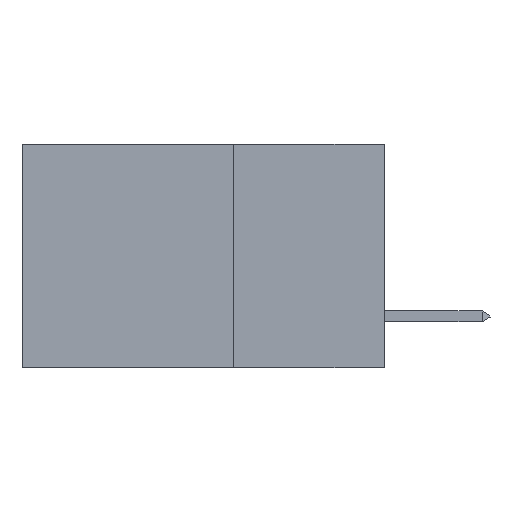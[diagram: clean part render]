
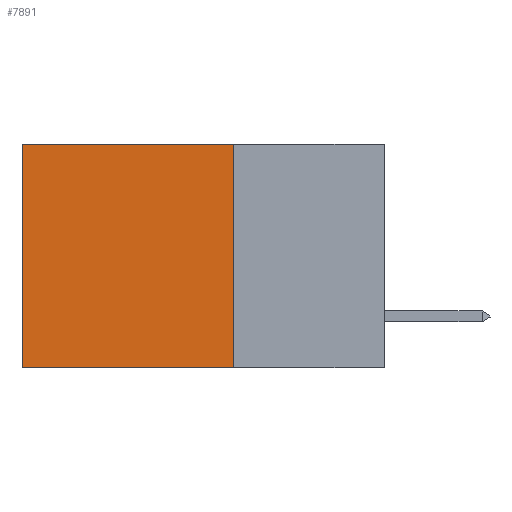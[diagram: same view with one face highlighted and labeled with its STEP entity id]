
A CAD part, left-side view. The second image highlights one B-rep face of the part: STEP entity #7891.
In plain terms, the highlighted planar face has unit normal (-1, 0, 0).
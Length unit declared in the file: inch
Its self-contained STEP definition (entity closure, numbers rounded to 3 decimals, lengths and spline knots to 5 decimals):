
#232 = ORIENTED_EDGE ( 'NONE', *, *, #8652, .T. ) ;
#660 = VERTEX_POINT ( 'NONE', #7267 ) ;
#1251 = EDGE_CURVE ( 'NONE', #660, #13368, #4878, .T. ) ;
#1410 = CARTESIAN_POINT ( 'NONE',  ( 0.2875, 0.25, 0. ) ) ;
#1565 = VECTOR ( 'NONE', #8554, 39.37008 ) ;
#3759 = ORIENTED_EDGE ( 'NONE', *, *, #11474, .T. ) ;
#3905 = VERTEX_POINT ( 'NONE', #6622 ) ;
#4120 = DIRECTION ( 'NONE',  ( 0., 0., -1. ) ) ;
#4446 = VECTOR ( 'NONE', #12484, 39.37008 ) ;
#4835 = LINE ( 'NONE', #7231, #4446 ) ;
#4878 = LINE ( 'NONE', #7297, #1565 ) ;
#4925 = VECTOR ( 'NONE', #14287, 39.37008 ) ;
#5098 = ORIENTED_EDGE ( 'NONE', *, *, #14194, .F. ) ;
#6283 = AXIS2_PLACEMENT_3D ( 'NONE', #7905, #9065, #4120 ) ;
#6622 = CARTESIAN_POINT ( 'NONE',  ( 0.2875, 0.25, 0. ) ) ;
#7231 = CARTESIAN_POINT ( 'NONE',  ( 0.2875, 0.25, 0. ) ) ;
#7267 = CARTESIAN_POINT ( 'NONE',  ( 0.2875, 0.25, -0.37 ) ) ;
#7297 = CARTESIAN_POINT ( 'NONE',  ( 0.2875, 0.25, -0.37 ) ) ;
#7891 = ADVANCED_FACE ( 'NONE', ( #11347 ), #15352, .F. ) ;
#7905 = CARTESIAN_POINT ( 'NONE',  ( 0.2875, 0.25, 0. ) ) ;
#8554 = DIRECTION ( 'NONE',  ( 0., 1., 0. ) ) ;
#8652 = EDGE_CURVE ( 'NONE', #3905, #8996, #4835, .T. ) ;
#8996 = VERTEX_POINT ( 'NONE', #14859 ) ;
#9065 = DIRECTION ( 'NONE',  ( 1., 0., 0. ) ) ;
#9902 = ORIENTED_EDGE ( 'NONE', *, *, #1251, .F. ) ;
#10791 = EDGE_LOOP ( 'NONE', ( #3759, #9902, #5098, #232 ) ) ;
#11347 = FACE_OUTER_BOUND ( 'NONE', #10791, .T. ) ;
#11474 = EDGE_CURVE ( 'NONE', #8996, #13368, #14932, .T. ) ;
#11504 = DIRECTION ( 'NONE',  ( 0., 0., -1. ) ) ;
#12474 = VECTOR ( 'NONE', #11504, 39.37008 ) ;
#12484 = DIRECTION ( 'NONE',  ( 0., 1., 0. ) ) ;
#13172 = CARTESIAN_POINT ( 'NONE',  ( 0.2875, 0.6, -0.37 ) ) ;
#13368 = VERTEX_POINT ( 'NONE', #13172 ) ;
#14182 = CARTESIAN_POINT ( 'NONE',  ( 0.2875, 0.6, 0. ) ) ;
#14194 = EDGE_CURVE ( 'NONE', #3905, #660, #15811, .T. ) ;
#14287 = DIRECTION ( 'NONE',  ( 0., 0., -1. ) ) ;
#14859 = CARTESIAN_POINT ( 'NONE',  ( 0.2875, 0.6, 0. ) ) ;
#14932 = LINE ( 'NONE', #14182, #4925 ) ;
#15352 = PLANE ( 'NONE',  #6283 ) ;
#15811 = LINE ( 'NONE', #1410, #12474 ) ;
